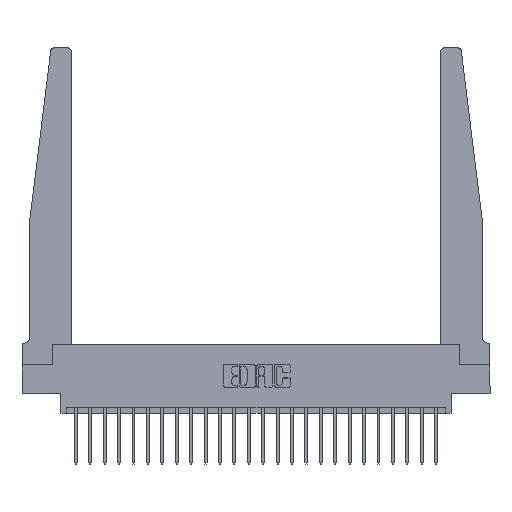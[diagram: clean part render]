
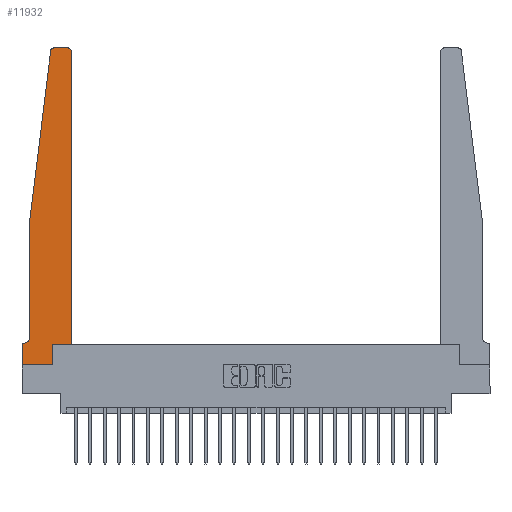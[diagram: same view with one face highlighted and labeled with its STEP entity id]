
A CAD part, top view. The second image highlights one B-rep face of the part: STEP entity #11932.
In plain terms, the highlighted planar face has unit normal (0, 0, 1).
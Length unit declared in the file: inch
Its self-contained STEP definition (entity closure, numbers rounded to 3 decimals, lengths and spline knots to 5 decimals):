
#194 = ORIENTED_EDGE ( 'NONE', *, *, #22904, .T. ) ;
#674 = CARTESIAN_POINT ( 'NONE',  ( 0., 0.1875, 0.37 ) ) ;
#1048 = DIRECTION ( 'NONE',  ( -0.122, -0.992, 0. ) ) ;
#1103 = DIRECTION ( 'NONE',  ( 0., -1., 0. ) ) ;
#1187 = CARTESIAN_POINT ( 'NONE',  ( 0., 0., 0.37 ) ) ;
#1359 = LINE ( 'NONE', #6655, #10670 ) ;
#1736 = PLANE ( 'NONE',  #6746 ) ;
#2009 = VECTOR ( 'NONE', #3741, 39.37008 ) ;
#2361 = CARTESIAN_POINT ( 'NONE',  ( 0.015, 0.1875, 0.37 ) ) ;
#3097 = EDGE_CURVE ( 'NONE', #19886, #5610, #4272, .T. ) ;
#3237 = EDGE_CURVE ( 'NONE', #17700, #19940, #1359, .T. ) ;
#3438 = VECTOR ( 'NONE', #18965, 39.37008 ) ;
#3533 = CARTESIAN_POINT ( 'NONE',  ( 0., 0.1875, 0.37 ) ) ;
#3609 = DIRECTION ( 'NONE',  ( 1., 0., 0. ) ) ;
#3660 = CARTESIAN_POINT ( 'NONE',  ( 0.2605, 0.18, 0.37 ) ) ;
#3741 = DIRECTION ( 'NONE',  ( 0., 1., 0. ) ) ;
#3800 = CARTESIAN_POINT ( 'NONE',  ( 0.425, 0.18, 0.37 ) ) ;
#3959 = CARTESIAN_POINT ( 'NONE',  ( 0.065, 1.25, 0.37 ) ) ;
#4272 = LINE ( 'NONE', #11905, #13567 ) ;
#4353 = CARTESIAN_POINT ( 'NONE',  ( 0.27653, 2.72, 0.37 ) ) ;
#4642 = CARTESIAN_POINT ( 'NONE',  ( 0.395, 2.75, 0.37 ) ) ;
#4805 = VECTOR ( 'NONE', #5680, 39.37008 ) ;
#4855 = DIRECTION ( 'NONE',  ( 1., 0., 0. ) ) ;
#5394 = DIRECTION ( 'NONE',  ( 0., 0., 1. ) ) ;
#5425 = EDGE_CURVE ( 'NONE', #19746, #17700, #11176, .T. ) ;
#5610 = VERTEX_POINT ( 'NONE', #10189 ) ;
#5680 = DIRECTION ( 'NONE',  ( 0., 1., 0. ) ) ;
#5712 = VERTEX_POINT ( 'NONE', #12284 ) ;
#5893 = EDGE_CURVE ( 'NONE', #9518, #19886, #7099, .T. ) ;
#6233 = AXIS2_PLACEMENT_3D ( 'NONE', #4353, #17399, #6238 ) ;
#6238 = DIRECTION ( 'NONE',  ( 1., 0., 0. ) ) ;
#6655 = CARTESIAN_POINT ( 'NONE',  ( 0., 0., 0.37 ) ) ;
#6746 = AXIS2_PLACEMENT_3D ( 'NONE', #3533, #14774, #3609 ) ;
#7029 = ORIENTED_EDGE ( 'NONE', *, *, #3097, .T. ) ;
#7033 = VECTOR ( 'NONE', #1048, 39.37008 ) ;
#7099 = CIRCLE ( 'NONE', #8822, 0.03 ) ;
#7135 = EDGE_CURVE ( 'NONE', #23731, #19746, #11112, .T. ) ;
#7310 = EDGE_CURVE ( 'NONE', #20827, #8619, #22495, .T. ) ;
#7331 = VERTEX_POINT ( 'NONE', #10388 ) ;
#7608 = ORIENTED_EDGE ( 'NONE', *, *, #7135, .T. ) ;
#8169 = DIRECTION ( 'NONE',  ( 1., 0., 0. ) ) ;
#8250 = ORIENTED_EDGE ( 'NONE', *, *, #16207, .T. ) ;
#8374 = CARTESIAN_POINT ( 'NONE',  ( 0.065, 1.25, 0.37 ) ) ;
#8619 = VERTEX_POINT ( 'NONE', #8374 ) ;
#8822 = AXIS2_PLACEMENT_3D ( 'NONE', #16565, #5394, #18438 ) ;
#8971 = LINE ( 'NONE', #3959, #3438 ) ;
#9518 = VERTEX_POINT ( 'NONE', #15116 ) ;
#9616 = EDGE_CURVE ( 'NONE', #5610, #20827, #23813, .T. ) ;
#9915 = CARTESIAN_POINT ( 'NONE',  ( 0.015, 0.2375, 0.37 ) ) ;
#9992 = VECTOR ( 'NONE', #8169, 39.37008 ) ;
#10075 = ORIENTED_EDGE ( 'NONE', *, *, #12874, .T. ) ;
#10189 = CARTESIAN_POINT ( 'NONE',  ( 0.27653, 2.75, 0.37 ) ) ;
#10388 = CARTESIAN_POINT ( 'NONE',  ( 0.2605, 0., 0.37 ) ) ;
#10670 = VECTOR ( 'NONE', #1103, 39.37008 ) ;
#10918 = CARTESIAN_POINT ( 'NONE',  ( 0.2605, 0.18, 0.37 ) ) ;
#11112 = CIRCLE ( 'NONE', #17438, 0.05 ) ;
#11176 = LINE ( 'NONE', #22756, #16759 ) ;
#11623 = EDGE_LOOP ( 'NONE', ( #7029, #16657, #22197, #21304, #7608, #19038, #17009, #21377, #8250, #194, #10075, #20592 ) ) ;
#11769 = DIRECTION ( 'NONE',  ( -1., 0., 0. ) ) ;
#11905 = CARTESIAN_POINT ( 'NONE',  ( 0.25, 2.75, 0.37 ) ) ;
#11932 = ADVANCED_FACE ( 'NONE', ( #22321 ), #1736, .T. ) ;
#12284 = CARTESIAN_POINT ( 'NONE',  ( 0.425, 0.18, 0.37 ) ) ;
#12467 = LINE ( 'NONE', #3660, #2009 ) ;
#12874 = EDGE_CURVE ( 'NONE', #5712, #9518, #14699, .T. ) ;
#13098 = VECTOR ( 'NONE', #4855, 39.37008 ) ;
#13567 = VECTOR ( 'NONE', #13788, 39.37008 ) ;
#13703 = CARTESIAN_POINT ( 'NONE',  ( 0.425, 0.18, 0.37 ) ) ;
#13788 = DIRECTION ( 'NONE',  ( -1., 0., 0. ) ) ;
#14045 = CARTESIAN_POINT ( 'NONE',  ( 0.065, 1.25, 0.37 ) ) ;
#14286 = LINE ( 'NONE', #1187, #13098 ) ;
#14699 = LINE ( 'NONE', #3800, #4805 ) ;
#14774 = DIRECTION ( 'NONE',  ( 0., 0., 1. ) ) ;
#14950 = LINE ( 'NONE', #13703, #9992 ) ;
#15116 = CARTESIAN_POINT ( 'NONE',  ( 0.425, 2.72, 0.37 ) ) ;
#15123 = EDGE_CURVE ( 'NONE', #19940, #7331, #14286, .T. ) ;
#15964 = CARTESIAN_POINT ( 'NONE',  ( 0., 0., 0.37 ) ) ;
#16207 = EDGE_CURVE ( 'NONE', #7331, #17956, #12467, .T. ) ;
#16565 = CARTESIAN_POINT ( 'NONE',  ( 0.395, 2.72, 0.37 ) ) ;
#16657 = ORIENTED_EDGE ( 'NONE', *, *, #9616, .T. ) ;
#16759 = VECTOR ( 'NONE', #19022, 39.37008 ) ;
#16864 = EDGE_CURVE ( 'NONE', #8619, #23731, #8971, .T. ) ;
#17009 = ORIENTED_EDGE ( 'NONE', *, *, #3237, .T. ) ;
#17399 = DIRECTION ( 'NONE',  ( 0., 0., 1. ) ) ;
#17438 = AXIS2_PLACEMENT_3D ( 'NONE', #9915, #22953, #11769 ) ;
#17700 = VERTEX_POINT ( 'NONE', #674 ) ;
#17932 = CARTESIAN_POINT ( 'NONE',  ( 0.065, 0.2375, 0.37 ) ) ;
#17956 = VERTEX_POINT ( 'NONE', #10918 ) ;
#18438 = DIRECTION ( 'NONE',  ( 1., 0., 0. ) ) ;
#18965 = DIRECTION ( 'NONE',  ( 0., -1., 0. ) ) ;
#19022 = DIRECTION ( 'NONE',  ( -1., 0., 0. ) ) ;
#19038 = ORIENTED_EDGE ( 'NONE', *, *, #5425, .T. ) ;
#19746 = VERTEX_POINT ( 'NONE', #2361 ) ;
#19886 = VERTEX_POINT ( 'NONE', #4642 ) ;
#19940 = VERTEX_POINT ( 'NONE', #15964 ) ;
#20592 = ORIENTED_EDGE ( 'NONE', *, *, #5893, .T. ) ;
#20827 = VERTEX_POINT ( 'NONE', #22763 ) ;
#21304 = ORIENTED_EDGE ( 'NONE', *, *, #16864, .T. ) ;
#21377 = ORIENTED_EDGE ( 'NONE', *, *, #15123, .T. ) ;
#22197 = ORIENTED_EDGE ( 'NONE', *, *, #7310, .T. ) ;
#22321 = FACE_OUTER_BOUND ( 'NONE', #11623, .T. ) ;
#22495 = LINE ( 'NONE', #14045, #7033 ) ;
#22756 = CARTESIAN_POINT ( 'NONE',  ( 0.065, 0.1875, 0.37 ) ) ;
#22763 = CARTESIAN_POINT ( 'NONE',  ( 0.24675, 2.72367, 0.37 ) ) ;
#22904 = EDGE_CURVE ( 'NONE', #17956, #5712, #14950, .T. ) ;
#22953 = DIRECTION ( 'NONE',  ( 0., 0., -1. ) ) ;
#23731 = VERTEX_POINT ( 'NONE', #17932 ) ;
#23813 = CIRCLE ( 'NONE', #6233, 0.03 ) ;
